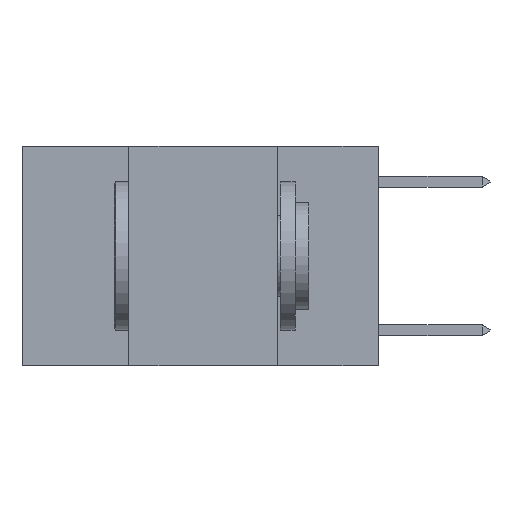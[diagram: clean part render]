
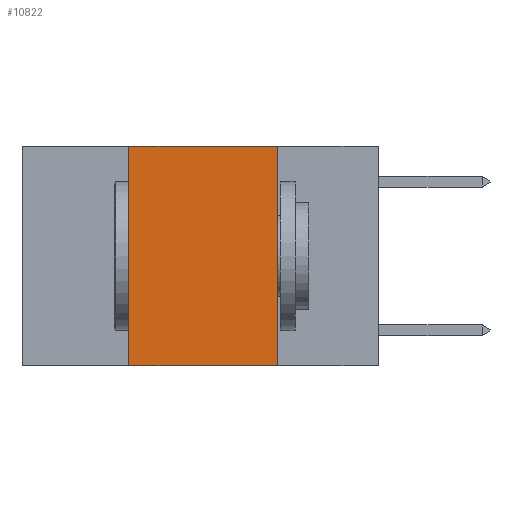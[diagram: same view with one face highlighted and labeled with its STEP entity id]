
A CAD part, left-side view. The second image highlights one B-rep face of the part: STEP entity #10822.
In plain terms, the highlighted planar face has unit normal (-1, 0, 0).
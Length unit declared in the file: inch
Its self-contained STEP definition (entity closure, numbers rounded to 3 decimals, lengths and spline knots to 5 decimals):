
#17 = ORIENTED_EDGE ( 'NONE', *, *, #18669, .F. ) ;
#197 = LINE ( 'NONE', #17562, #22544 ) ;
#697 = ORIENTED_EDGE ( 'NONE', *, *, #6357, .T. ) ;
#4658 = DIRECTION ( 'NONE',  ( 1., 0., 0. ) ) ;
#4945 = CARTESIAN_POINT ( 'NONE',  ( 0., 0.6, 0. ) ) ;
#5055 = ORIENTED_EDGE ( 'NONE', *, *, #12509, .F. ) ;
#5065 = CARTESIAN_POINT ( 'NONE',  ( 0., 0.42, 0. ) ) ;
#5419 = LINE ( 'NONE', #21227, #20767 ) ;
#6357 = EDGE_CURVE ( 'NONE', #13349, #7890, #21329, .T. ) ;
#6867 = FACE_OUTER_BOUND ( 'NONE', #16970, .T. ) ;
#7890 = VERTEX_POINT ( 'NONE', #29219 ) ;
#8929 = CARTESIAN_POINT ( 'NONE',  ( 0., 0.42, 0. ) ) ;
#10008 = DIRECTION ( 'NONE',  ( 0., -1., 0. ) ) ;
#10822 = ADVANCED_FACE ( 'NONE', ( #6867 ), #24913, .F. ) ;
#12049 = DIRECTION ( 'NONE',  ( 0., 0., -1. ) ) ;
#12509 = EDGE_CURVE ( 'NONE', #13349, #26143, #26664, .T. ) ;
#13349 = VERTEX_POINT ( 'NONE', #14467 ) ;
#14416 = CARTESIAN_POINT ( 'NONE',  ( 0., 0.6, -0.37 ) ) ;
#14467 = CARTESIAN_POINT ( 'NONE',  ( 0., 0.42, -0.37 ) ) ;
#14481 = AXIS2_PLACEMENT_3D ( 'NONE', #4945, #4658, #12049 ) ;
#16805 = VECTOR ( 'NONE', #10008, 39.37008 ) ;
#16970 = EDGE_LOOP ( 'NONE', ( #17586, #17, #5055, #697 ) ) ;
#17562 = CARTESIAN_POINT ( 'NONE',  ( 0., 0.17, 0. ) ) ;
#17586 = ORIENTED_EDGE ( 'NONE', *, *, #25640, .F. ) ;
#18669 = EDGE_CURVE ( 'NONE', #26143, #24415, #5419, .T. ) ;
#19830 = DIRECTION ( 'NONE',  ( 0., 0., 1. ) ) ;
#20767 = VECTOR ( 'NONE', #25388, 39.37008 ) ;
#21227 = CARTESIAN_POINT ( 'NONE',  ( 0., 0.6, 0. ) ) ;
#21329 = LINE ( 'NONE', #14416, #16805 ) ;
#22544 = VECTOR ( 'NONE', #26604, 39.37008 ) ;
#23116 = CARTESIAN_POINT ( 'NONE',  ( 0., 0.17, 0. ) ) ;
#24415 = VERTEX_POINT ( 'NONE', #23116 ) ;
#24913 = PLANE ( 'NONE',  #14481 ) ;
#25388 = DIRECTION ( 'NONE',  ( 0., -1., 0. ) ) ;
#25640 = EDGE_CURVE ( 'NONE', #24415, #7890, #197, .T. ) ;
#26143 = VERTEX_POINT ( 'NONE', #5065 ) ;
#26470 = VECTOR ( 'NONE', #19830, 39.37008 ) ;
#26604 = DIRECTION ( 'NONE',  ( 0., 0., -1. ) ) ;
#26664 = LINE ( 'NONE', #8929, #26470 ) ;
#29219 = CARTESIAN_POINT ( 'NONE',  ( 0., 0.17, -0.37 ) ) ;
